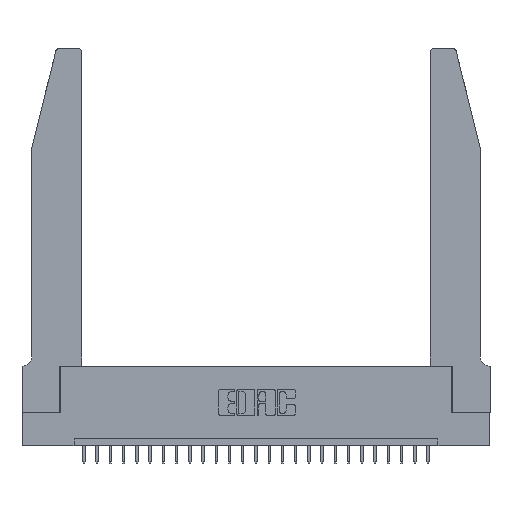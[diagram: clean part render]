
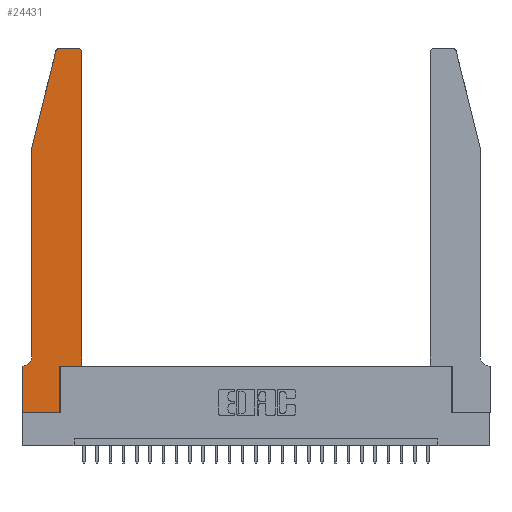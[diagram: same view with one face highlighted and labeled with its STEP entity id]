
A CAD part, top view. The second image highlights one B-rep face of the part: STEP entity #24431.
In plain terms, the highlighted planar face has unit normal (0, 0, 1).
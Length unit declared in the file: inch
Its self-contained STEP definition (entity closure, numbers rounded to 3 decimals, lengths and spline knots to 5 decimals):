
#381 = CARTESIAN_POINT ( 'NONE',  ( 0., 0., 0.37 ) ) ;
#642 = VERTEX_POINT ( 'NONE', #11952 ) ;
#788 = CARTESIAN_POINT ( 'NONE',  ( 0., 0.35, 0.37 ) ) ;
#884 = CARTESIAN_POINT ( 'NONE',  ( 0.0755, 2., 0.37 ) ) ;
#1182 = ORIENTED_EDGE ( 'NONE', *, *, #23753, .T. ) ;
#1235 = VERTEX_POINT ( 'NONE', #20559 ) ;
#2377 = CARTESIAN_POINT ( 'NONE',  ( 0.2865, 0.35, 0.37 ) ) ;
#2570 = VECTOR ( 'NONE', #19743, 39.37008 ) ;
#2642 = EDGE_CURVE ( 'NONE', #642, #3690, #26050, .T. ) ;
#2824 = ORIENTED_EDGE ( 'NONE', *, *, #17391, .T. ) ;
#2841 = EDGE_CURVE ( 'NONE', #4708, #24745, #21393, .T. ) ;
#3690 = VERTEX_POINT ( 'NONE', #7946 ) ;
#4580 = DIRECTION ( 'NONE',  ( -1., 0., 0. ) ) ;
#4708 = VERTEX_POINT ( 'NONE', #23360 ) ;
#4735 = EDGE_CURVE ( 'NONE', #22373, #25343, #21199, .T. ) ;
#4751 = CARTESIAN_POINT ( 'NONE',  ( 0., 0.35, 0.37 ) ) ;
#4762 = CARTESIAN_POINT ( 'NONE',  ( 0., 0., 0.37 ) ) ;
#5022 = CARTESIAN_POINT ( 'NONE',  ( 0.284, 2.72, 0.37 ) ) ;
#5409 = CARTESIAN_POINT ( 'NONE',  ( 0.284, 2.75, 0.37 ) ) ;
#5611 = DIRECTION ( 'NONE',  ( 0., 0., 1. ) ) ;
#5754 = CIRCLE ( 'NONE', #19787, 0.07 ) ;
#6118 = ORIENTED_EDGE ( 'NONE', *, *, #13041, .T. ) ;
#6301 = ORIENTED_EDGE ( 'NONE', *, *, #2841, .T. ) ;
#6538 = VERTEX_POINT ( 'NONE', #23427 ) ;
#6568 = DIRECTION ( 'NONE',  ( 1., 0., 0. ) ) ;
#6691 = DIRECTION ( 'NONE',  ( 0., 0., 1. ) ) ;
#6757 = DIRECTION ( 'NONE',  ( 0., 1., 0. ) ) ;
#7071 = VECTOR ( 'NONE', #4580, 39.37008 ) ;
#7315 = ORIENTED_EDGE ( 'NONE', *, *, #16239, .T. ) ;
#7946 = CARTESIAN_POINT ( 'NONE',  ( 0.4205, 2.75, 0.37 ) ) ;
#8335 = EDGE_CURVE ( 'NONE', #1235, #14777, #10352, .T. ) ;
#8593 = ORIENTED_EDGE ( 'NONE', *, *, #9147, .T. ) ;
#8627 = CARTESIAN_POINT ( 'NONE',  ( 0.4505, 0.35, 0.37 ) ) ;
#8924 = VECTOR ( 'NONE', #6568, 39.37008 ) ;
#8976 = DIRECTION ( 'NONE',  ( 0., 1., 0. ) ) ;
#9147 = EDGE_CURVE ( 'NONE', #14777, #24841, #25083, .T. ) ;
#9858 = LINE ( 'NONE', #18237, #17504 ) ;
#10123 = AXIS2_PLACEMENT_3D ( 'NONE', #5022, #25778, #19459 ) ;
#10352 = LINE ( 'NONE', #22450, #17805 ) ;
#10644 = DIRECTION ( 'NONE',  ( 1., 0., 0. ) ) ;
#10668 = VECTOR ( 'NONE', #6757, 39.37008 ) ;
#11029 = LINE ( 'NONE', #2377, #14497 ) ;
#11208 = ORIENTED_EDGE ( 'NONE', *, *, #17700, .T. ) ;
#11910 = CARTESIAN_POINT ( 'NONE',  ( 0.0055, 0.42, 0.37 ) ) ;
#11952 = CARTESIAN_POINT ( 'NONE',  ( 0.4505, 2.72, 0.37 ) ) ;
#12193 = CARTESIAN_POINT ( 'NONE',  ( 0.0755, 2., 0.37 ) ) ;
#12509 = CARTESIAN_POINT ( 'NONE',  ( 0.0055, 0.35, 0.37 ) ) ;
#12671 = CARTESIAN_POINT ( 'NONE',  ( 0.4505, 0.35, 0.37 ) ) ;
#12855 = FACE_OUTER_BOUND ( 'NONE', #24764, .T. ) ;
#13041 = EDGE_CURVE ( 'NONE', #3690, #24524, #9858, .T. ) ;
#13286 = ORIENTED_EDGE ( 'NONE', *, *, #8335, .T. ) ;
#13332 = EDGE_CURVE ( 'NONE', #20919, #6538, #23548, .T. ) ;
#13397 = VECTOR ( 'NONE', #18403, 39.37008 ) ;
#13611 = ORIENTED_EDGE ( 'NONE', *, *, #19169, .T. ) ;
#14462 = ORIENTED_EDGE ( 'NONE', *, *, #4735, .T. ) ;
#14497 = VECTOR ( 'NONE', #8976, 39.37008 ) ;
#14671 = DIRECTION ( 'NONE',  ( 0., -1., 0. ) ) ;
#14777 = VERTEX_POINT ( 'NONE', #884 ) ;
#14890 = CARTESIAN_POINT ( 'NONE',  ( 0.0755, 0.35, 0.37 ) ) ;
#16150 = DIRECTION ( 'NONE',  ( -0.239, -0.971, 0. ) ) ;
#16239 = EDGE_CURVE ( 'NONE', #6538, #4708, #11029, .T. ) ;
#16334 = DIRECTION ( 'NONE',  ( 0., 0., -1. ) ) ;
#16551 = VECTOR ( 'NONE', #14671, 39.37008 ) ;
#16796 = LINE ( 'NONE', #12671, #10668 ) ;
#17349 = CARTESIAN_POINT ( 'NONE',  ( 0.0755, 0.42, 0.37 ) ) ;
#17391 = EDGE_CURVE ( 'NONE', #24841, #22373, #5754, .T. ) ;
#17504 = VECTOR ( 'NONE', #20590, 39.37008 ) ;
#17700 = EDGE_CURVE ( 'NONE', #24524, #1235, #21544, .T. ) ;
#17805 = VECTOR ( 'NONE', #16150, 39.37008 ) ;
#18237 = CARTESIAN_POINT ( 'NONE',  ( 0.2605, 2.75, 0.37 ) ) ;
#18403 = DIRECTION ( 'NONE',  ( 0., -1., 0. ) ) ;
#18676 = LINE ( 'NONE', #26786, #13397 ) ;
#19169 = EDGE_CURVE ( 'NONE', #24745, #642, #16796, .T. ) ;
#19459 = DIRECTION ( 'NONE',  ( 1., 0., 0. ) ) ;
#19511 = ORIENTED_EDGE ( 'NONE', *, *, #13332, .T. ) ;
#19651 = ORIENTED_EDGE ( 'NONE', *, *, #2642, .T. ) ;
#19743 = DIRECTION ( 'NONE',  ( 1., 0., 0. ) ) ;
#19787 = AXIS2_PLACEMENT_3D ( 'NONE', #11910, #16334, #22636 ) ;
#20303 = DIRECTION ( 'NONE',  ( 1., 0., 0. ) ) ;
#20559 = CARTESIAN_POINT ( 'NONE',  ( 0.25487, 2.72718, 0.37 ) ) ;
#20590 = DIRECTION ( 'NONE',  ( -1., 0., 0. ) ) ;
#20919 = VERTEX_POINT ( 'NONE', #381 ) ;
#20944 = CARTESIAN_POINT ( 'NONE',  ( 0.4505, 0.35, 0.37 ) ) ;
#21199 = LINE ( 'NONE', #14890, #7071 ) ;
#21393 = LINE ( 'NONE', #8627, #8924 ) ;
#21544 = CIRCLE ( 'NONE', #10123, 0.03 ) ;
#21650 = PLANE ( 'NONE',  #22627 ) ;
#22373 = VERTEX_POINT ( 'NONE', #12509 ) ;
#22450 = CARTESIAN_POINT ( 'NONE',  ( 0.0755, 2., 0.37 ) ) ;
#22627 = AXIS2_PLACEMENT_3D ( 'NONE', #4751, #6691, #10644 ) ;
#22636 = DIRECTION ( 'NONE',  ( -1., 0., 0. ) ) ;
#23360 = CARTESIAN_POINT ( 'NONE',  ( 0.2865, 0.35, 0.37 ) ) ;
#23427 = CARTESIAN_POINT ( 'NONE',  ( 0.2865, 0., 0.37 ) ) ;
#23548 = LINE ( 'NONE', #4762, #2570 ) ;
#23753 = EDGE_CURVE ( 'NONE', #25343, #20919, #18676, .T. ) ;
#24269 = CARTESIAN_POINT ( 'NONE',  ( 0.4205, 2.72, 0.37 ) ) ;
#24280 = AXIS2_PLACEMENT_3D ( 'NONE', #24269, #5611, #20303 ) ;
#24431 = ADVANCED_FACE ( 'NONE', ( #12855 ), #21650, .T. ) ;
#24524 = VERTEX_POINT ( 'NONE', #5409 ) ;
#24745 = VERTEX_POINT ( 'NONE', #20944 ) ;
#24764 = EDGE_LOOP ( 'NONE', ( #6118, #11208, #13286, #8593, #2824, #14462, #1182, #19511, #7315, #6301, #13611, #19651 ) ) ;
#24841 = VERTEX_POINT ( 'NONE', #17349 ) ;
#25083 = LINE ( 'NONE', #12193, #16551 ) ;
#25343 = VERTEX_POINT ( 'NONE', #788 ) ;
#25778 = DIRECTION ( 'NONE',  ( 0., 0., 1. ) ) ;
#26050 = CIRCLE ( 'NONE', #24280, 0.03 ) ;
#26786 = CARTESIAN_POINT ( 'NONE',  ( 0., 0., 0.37 ) ) ;
